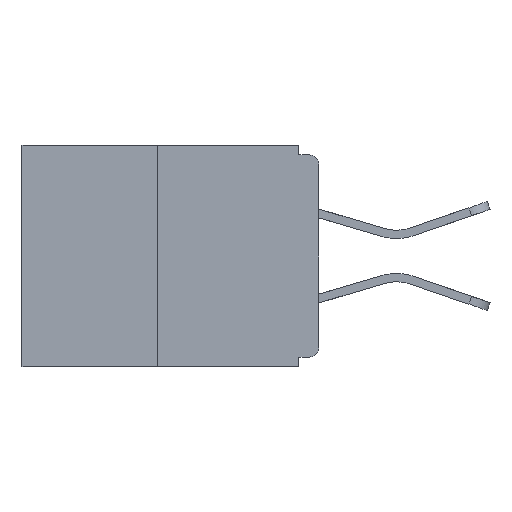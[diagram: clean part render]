
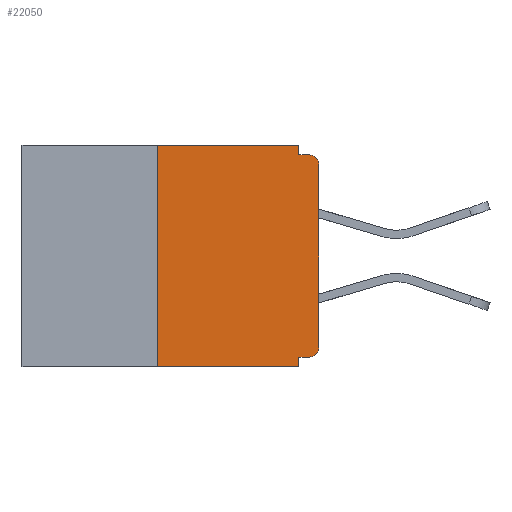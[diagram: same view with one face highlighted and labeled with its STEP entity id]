
A CAD part, left-side view. The second image highlights one B-rep face of the part: STEP entity #22050.
In plain terms, the highlighted planar face has unit normal (-1, 0, 0).
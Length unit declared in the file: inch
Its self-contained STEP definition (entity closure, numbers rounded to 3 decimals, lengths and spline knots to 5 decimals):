
#304 = VECTOR ( 'NONE', #14744, 39.37008 ) ;
#423 = ORIENTED_EDGE ( 'NONE', *, *, #18906, .F. ) ;
#504 = VECTOR ( 'NONE', #20425, 39.37008 ) ;
#649 = VECTOR ( 'NONE', #1483, 39.37008 ) ;
#997 = CARTESIAN_POINT ( 'NONE',  ( 0., 0.031, 0. ) ) ;
#1113 = DIRECTION ( 'NONE',  ( -1., 0., 0. ) ) ;
#1296 = VERTEX_POINT ( 'NONE', #21521 ) ;
#1483 = DIRECTION ( 'NONE',  ( 0., -1., 0. ) ) ;
#1974 = CARTESIAN_POINT ( 'NONE',  ( 0., 0., -0.03 ) ) ;
#2293 = VERTEX_POINT ( 'NONE', #16660 ) ;
#2525 = CARTESIAN_POINT ( 'NONE',  ( 0., 0.46, -0.343 ) ) ;
#2751 = VERTEX_POINT ( 'NONE', #4765 ) ;
#2863 = LINE ( 'NONE', #9786, #6321 ) ;
#3033 = DIRECTION ( 'NONE',  ( 0., 0., -1. ) ) ;
#3356 = LINE ( 'NONE', #13949, #18737 ) ;
#3592 = ORIENTED_EDGE ( 'NONE', *, *, #11818, .F. ) ;
#3892 = EDGE_CURVE ( 'NONE', #1296, #2293, #17072, .T. ) ;
#4024 = CARTESIAN_POINT ( 'NONE',  ( 0., 0.25, 0. ) ) ;
#4476 = EDGE_CURVE ( 'NONE', #9508, #22321, #9587, .T. ) ;
#4765 = CARTESIAN_POINT ( 'NONE',  ( 0., 0.031, -0.328 ) ) ;
#4827 = AXIS2_PLACEMENT_3D ( 'NONE', #19781, #1113, #3033 ) ;
#5241 = EDGE_CURVE ( 'NONE', #16143, #22321, #16853, .T. ) ;
#5662 = VERTEX_POINT ( 'NONE', #12446 ) ;
#5698 = LINE ( 'NONE', #10937, #14602 ) ;
#5869 = EDGE_CURVE ( 'NONE', #13729, #2751, #8656, .T. ) ;
#6062 = CIRCLE ( 'NONE', #19152, 0.015 ) ;
#6186 = EDGE_CURVE ( 'NONE', #9044, #16143, #2863, .T. ) ;
#6242 = ORIENTED_EDGE ( 'NONE', *, *, #5869, .F. ) ;
#6321 = VECTOR ( 'NONE', #16754, 39.37008 ) ;
#6833 = EDGE_CURVE ( 'NONE', #12259, #9508, #3356, .T. ) ;
#8370 = CARTESIAN_POINT ( 'NONE',  ( 0., 0.46, 0. ) ) ;
#8627 = ORIENTED_EDGE ( 'NONE', *, *, #6833, .F. ) ;
#8655 = ORIENTED_EDGE ( 'NONE', *, *, #22493, .F. ) ;
#8656 = LINE ( 'NONE', #12084, #504 ) ;
#9044 = VERTEX_POINT ( 'NONE', #14955 ) ;
#9181 = CARTESIAN_POINT ( 'NONE',  ( 0., 0.015, -0.313 ) ) ;
#9508 = VERTEX_POINT ( 'NONE', #13082 ) ;
#9587 = LINE ( 'NONE', #20313, #304 ) ;
#9786 = CARTESIAN_POINT ( 'NONE',  ( 0., 0., 0. ) ) ;
#9850 = CARTESIAN_POINT ( 'NONE',  ( 0., 0.015, -0.015 ) ) ;
#10624 = DIRECTION ( 'NONE',  ( 0., -1., 0. ) ) ;
#10937 = CARTESIAN_POINT ( 'NONE',  ( 0., 0.031, -0.343 ) ) ;
#11814 = FACE_OUTER_BOUND ( 'NONE', #22183, .T. ) ;
#11818 = EDGE_CURVE ( 'NONE', #1296, #5662, #19754, .T. ) ;
#11834 = ORIENTED_EDGE ( 'NONE', *, *, #15343, .T. ) ;
#12084 = CARTESIAN_POINT ( 'NONE',  ( 0., 0., -0.328 ) ) ;
#12259 = VERTEX_POINT ( 'NONE', #997 ) ;
#12279 = ORIENTED_EDGE ( 'NONE', *, *, #3892, .T. ) ;
#12446 = CARTESIAN_POINT ( 'NONE',  ( 0., 0.25, 0. ) ) ;
#12481 = VECTOR ( 'NONE', #10624, 39.37008 ) ;
#13082 = CARTESIAN_POINT ( 'NONE',  ( 0., 0.031, -0.015 ) ) ;
#13292 = PLANE ( 'NONE',  #19435 ) ;
#13636 = DIRECTION ( 'NONE',  ( 0., 0., -1. ) ) ;
#13729 = VERTEX_POINT ( 'NONE', #18944 ) ;
#13949 = CARTESIAN_POINT ( 'NONE',  ( 0., 0.031, 0. ) ) ;
#14327 = DIRECTION ( 'NONE',  ( -1., 0., 0. ) ) ;
#14602 = VECTOR ( 'NONE', #16082, 39.37008 ) ;
#14744 = DIRECTION ( 'NONE',  ( 0., -1., 0. ) ) ;
#14955 = CARTESIAN_POINT ( 'NONE',  ( 0., 0., -0.313 ) ) ;
#15343 = EDGE_CURVE ( 'NONE', #13729, #9044, #6062, .T. ) ;
#16082 = DIRECTION ( 'NONE',  ( 0., 0., -1. ) ) ;
#16143 = VERTEX_POINT ( 'NONE', #1974 ) ;
#16660 = CARTESIAN_POINT ( 'NONE',  ( 0., 0.031, -0.343 ) ) ;
#16754 = DIRECTION ( 'NONE',  ( 0., 0., 1. ) ) ;
#16853 = CIRCLE ( 'NONE', #4827, 0.015 ) ;
#17072 = LINE ( 'NONE', #2525, #649 ) ;
#17934 = DIRECTION ( 'NONE',  ( 0., 0., 1. ) ) ;
#18737 = VECTOR ( 'NONE', #20906, 39.37008 ) ;
#18906 = EDGE_CURVE ( 'NONE', #2751, #2293, #5698, .T. ) ;
#18944 = CARTESIAN_POINT ( 'NONE',  ( 0., 0.015, -0.328 ) ) ;
#19152 = AXIS2_PLACEMENT_3D ( 'NONE', #9181, #14327, #19907 ) ;
#19183 = CARTESIAN_POINT ( 'NONE',  ( 0., 0.46, 0. ) ) ;
#19214 = ORIENTED_EDGE ( 'NONE', *, *, #5241, .T. ) ;
#19435 = AXIS2_PLACEMENT_3D ( 'NONE', #8370, #22303, #13636 ) ;
#19754 = LINE ( 'NONE', #4024, #20934 ) ;
#19781 = CARTESIAN_POINT ( 'NONE',  ( 0., 0.015, -0.03 ) ) ;
#19907 = DIRECTION ( 'NONE',  ( 0., 0., -1. ) ) ;
#19966 = ORIENTED_EDGE ( 'NONE', *, *, #6186, .T. ) ;
#20313 = CARTESIAN_POINT ( 'NONE',  ( 0., 0., -0.015 ) ) ;
#20425 = DIRECTION ( 'NONE',  ( 0., 1., 0. ) ) ;
#20906 = DIRECTION ( 'NONE',  ( 0., 0., -1. ) ) ;
#20934 = VECTOR ( 'NONE', #17934, 39.37008 ) ;
#21340 = LINE ( 'NONE', #19183, #12481 ) ;
#21521 = CARTESIAN_POINT ( 'NONE',  ( 0., 0.25, -0.343 ) ) ;
#21881 = ORIENTED_EDGE ( 'NONE', *, *, #4476, .F. ) ;
#22050 = ADVANCED_FACE ( 'NONE', ( #11814 ), #13292, .F. ) ;
#22183 = EDGE_LOOP ( 'NONE', ( #8655, #3592, #12279, #423, #6242, #11834, #19966, #19214, #21881, #8627 ) ) ;
#22303 = DIRECTION ( 'NONE',  ( 1., 0., 0. ) ) ;
#22321 = VERTEX_POINT ( 'NONE', #9850 ) ;
#22493 = EDGE_CURVE ( 'NONE', #5662, #12259, #21340, .T. ) ;
